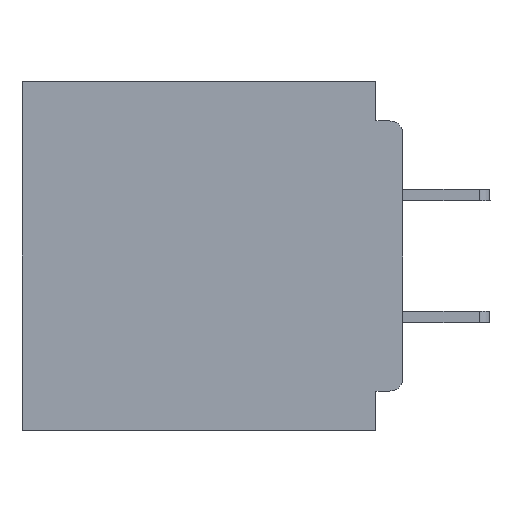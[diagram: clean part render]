
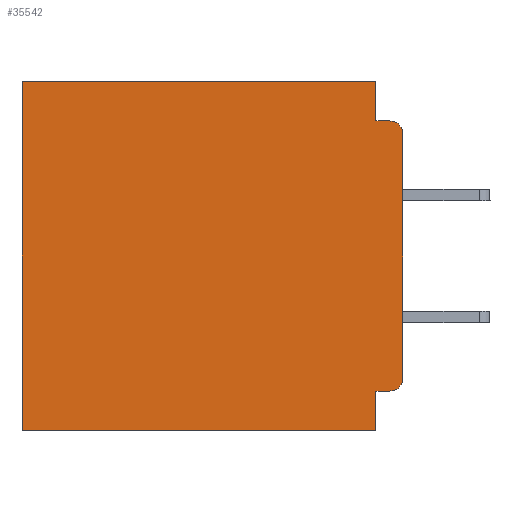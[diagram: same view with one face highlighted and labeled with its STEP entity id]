
A CAD part, left-side view. The second image highlights one B-rep face of the part: STEP entity #35542.
In plain terms, the highlighted planar face has unit normal (-1, 0, 0).
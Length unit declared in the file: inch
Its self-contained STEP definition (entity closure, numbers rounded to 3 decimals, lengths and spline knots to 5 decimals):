
#695 = VERTEX_POINT ( 'NONE', #63557 ) ;
#962 = AXIS2_PLACEMENT_3D ( 'NONE', #28157, #38132, #8352 ) ;
#2301 = VERTEX_POINT ( 'NONE', #27987 ) ;
#2507 = DIRECTION ( 'NONE',  ( -1., 0., 0. ) ) ;
#4441 = VECTOR ( 'NONE', #9557, 39.37008 ) ;
#4535 = LINE ( 'NONE', #64204, #44315 ) ;
#7305 = VECTOR ( 'NONE', #11314, 39.37008 ) ;
#7365 = EDGE_CURVE ( 'NONE', #61656, #56737, #59582, .T. ) ;
#8352 = DIRECTION ( 'NONE',  ( 0., 0., -1. ) ) ;
#8633 = ORIENTED_EDGE ( 'NONE', *, *, #14465, .T. ) ;
#9557 = DIRECTION ( 'NONE',  ( 0., 0., -1. ) ) ;
#9564 = DIRECTION ( 'NONE',  ( 0., 0., -1. ) ) ;
#11314 = DIRECTION ( 'NONE',  ( 0., 1., 0. ) ) ;
#12029 = EDGE_CURVE ( 'NONE', #44387, #21400, #47541, .T. ) ;
#13053 = ORIENTED_EDGE ( 'NONE', *, *, #44374, .T. ) ;
#13857 = ORIENTED_EDGE ( 'NONE', *, *, #12029, .F. ) ;
#14465 = EDGE_CURVE ( 'NONE', #2301, #15732, #23116, .T. ) ;
#15298 = FACE_OUTER_BOUND ( 'NONE', #39384, .T. ) ;
#15562 = CIRCLE ( 'NONE', #34005, 0.015 ) ;
#15732 = VERTEX_POINT ( 'NONE', #41242 ) ;
#17777 = LINE ( 'NONE', #59080, #4441 ) ;
#20238 = VERTEX_POINT ( 'NONE', #37333 ) ;
#20569 = LINE ( 'NONE', #36075, #7305 ) ;
#21119 = VECTOR ( 'NONE', #9564, 39.37008 ) ;
#21151 = LINE ( 'NONE', #50939, #46037 ) ;
#21400 = VERTEX_POINT ( 'NONE', #61084 ) ;
#23116 = CIRCLE ( 'NONE', #64296, 0.015 ) ;
#23600 = EDGE_CURVE ( 'NONE', #695, #55278, #4535, .T. ) ;
#24273 = VECTOR ( 'NONE', #61895, 39.37008 ) ;
#25763 = VECTOR ( 'NONE', #46278, 39.37008 ) ;
#26646 = DIRECTION ( 'NONE',  ( -1., 0., 0. ) ) ;
#27169 = ORIENTED_EDGE ( 'NONE', *, *, #49033, .F. ) ;
#27987 = CARTESIAN_POINT ( 'NONE',  ( 0.3, 0.015, -0.355 ) ) ;
#28157 = CARTESIAN_POINT ( 'NONE',  ( 0.3, 0., -0.4 ) ) ;
#29336 = CARTESIAN_POINT ( 'NONE',  ( 0.3, 0.031, -0.4 ) ) ;
#31262 = CARTESIAN_POINT ( 'NONE',  ( 0.3, 0., -0.4 ) ) ;
#32372 = DIRECTION ( 'NONE',  ( 0., 1., 0. ) ) ;
#32448 = CARTESIAN_POINT ( 'NONE',  ( 0.3, 0.015, -0.06 ) ) ;
#32581 = CARTESIAN_POINT ( 'NONE',  ( 0.3, 0., 0. ) ) ;
#34005 = AXIS2_PLACEMENT_3D ( 'NONE', #32448, #2507, #37438 ) ;
#35542 = ADVANCED_FACE ( 'NONE', ( #15298 ), #57878, .F. ) ;
#36075 = CARTESIAN_POINT ( 'NONE',  ( 0.3, 0., -0.4 ) ) ;
#36552 = EDGE_CURVE ( 'NONE', #21400, #20238, #20569, .T. ) ;
#37333 = CARTESIAN_POINT ( 'NONE',  ( 0.3, 0.437, -0.4 ) ) ;
#37402 = LINE ( 'NONE', #31262, #25763 ) ;
#37438 = DIRECTION ( 'NONE',  ( 0., 0., -1. ) ) ;
#37758 = CARTESIAN_POINT ( 'NONE',  ( 0.3, 0., -0.06 ) ) ;
#38132 = DIRECTION ( 'NONE',  ( 1., 0., 0. ) ) ;
#39384 = EDGE_LOOP ( 'NONE', ( #53035, #63198, #39587, #41722, #46309, #13053, #50822, #13857, #27169, #8633 ) ) ;
#39587 = ORIENTED_EDGE ( 'NONE', *, *, #23600, .F. ) ;
#40072 = CARTESIAN_POINT ( 'NONE',  ( 0.3, 0.015, -0.045 ) ) ;
#41242 = CARTESIAN_POINT ( 'NONE',  ( 0.3, 0., -0.34 ) ) ;
#41722 = ORIENTED_EDGE ( 'NONE', *, *, #56326, .F. ) ;
#44315 = VECTOR ( 'NONE', #49226, 39.37008 ) ;
#44374 = EDGE_CURVE ( 'NONE', #56737, #20238, #21151, .T. ) ;
#44387 = VERTEX_POINT ( 'NONE', #61156 ) ;
#46037 = VECTOR ( 'NONE', #55923, 39.37008 ) ;
#46278 = DIRECTION ( 'NONE',  ( 0., 0., -1. ) ) ;
#46309 = ORIENTED_EDGE ( 'NONE', *, *, #7365, .T. ) ;
#47541 = LINE ( 'NONE', #29336, #21119 ) ;
#49033 = EDGE_CURVE ( 'NONE', #2301, #44387, #63921, .T. ) ;
#49226 = DIRECTION ( 'NONE',  ( 0., -1., 0. ) ) ;
#50263 = EDGE_CURVE ( 'NONE', #54452, #55278, #15562, .T. ) ;
#50822 = ORIENTED_EDGE ( 'NONE', *, *, #36552, .F. ) ;
#50939 = CARTESIAN_POINT ( 'NONE',  ( 0.3, 0.437, -0.4 ) ) ;
#53035 = ORIENTED_EDGE ( 'NONE', *, *, #54237, .F. ) ;
#54237 = EDGE_CURVE ( 'NONE', #54452, #15732, #37402, .T. ) ;
#54452 = VERTEX_POINT ( 'NONE', #37758 ) ;
#55278 = VERTEX_POINT ( 'NONE', #40072 ) ;
#55923 = DIRECTION ( 'NONE',  ( 0., 0., -1. ) ) ;
#56326 = EDGE_CURVE ( 'NONE', #61656, #695, #17777, .T. ) ;
#56350 = CARTESIAN_POINT ( 'NONE',  ( 0.3, 0.015, -0.34 ) ) ;
#56737 = VERTEX_POINT ( 'NONE', #57271 ) ;
#56871 = CARTESIAN_POINT ( 'NONE',  ( 0.3, 0., -0.355 ) ) ;
#57271 = CARTESIAN_POINT ( 'NONE',  ( 0.3, 0.437, 0. ) ) ;
#57878 = PLANE ( 'NONE',  #962 ) ;
#58014 = VECTOR ( 'NONE', #32372, 39.37008 ) ;
#59080 = CARTESIAN_POINT ( 'NONE',  ( 0.3, 0.031, 0. ) ) ;
#59582 = LINE ( 'NONE', #32581, #58014 ) ;
#61084 = CARTESIAN_POINT ( 'NONE',  ( 0.3, 0.031, -0.4 ) ) ;
#61156 = CARTESIAN_POINT ( 'NONE',  ( 0.3, 0.031, -0.355 ) ) ;
#61395 = DIRECTION ( 'NONE',  ( 0., 0., -1. ) ) ;
#61656 = VERTEX_POINT ( 'NONE', #63063 ) ;
#61895 = DIRECTION ( 'NONE',  ( 0., 1., 0. ) ) ;
#63063 = CARTESIAN_POINT ( 'NONE',  ( 0.3, 0.031, 0. ) ) ;
#63198 = ORIENTED_EDGE ( 'NONE', *, *, #50263, .T. ) ;
#63557 = CARTESIAN_POINT ( 'NONE',  ( 0.3, 0.031, -0.045 ) ) ;
#63921 = LINE ( 'NONE', #56871, #24273 ) ;
#64204 = CARTESIAN_POINT ( 'NONE',  ( 0.3, 0., -0.045 ) ) ;
#64296 = AXIS2_PLACEMENT_3D ( 'NONE', #56350, #26646, #61395 ) ;
